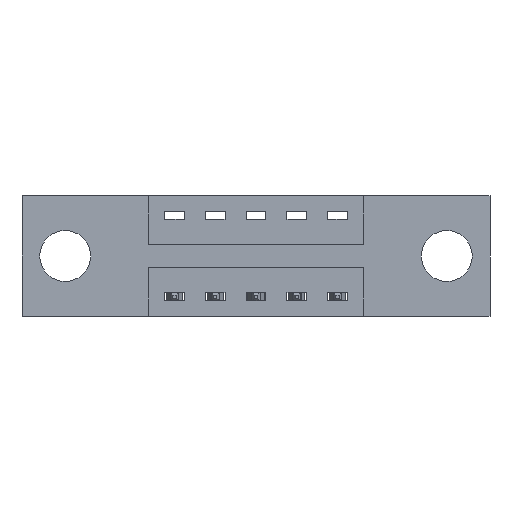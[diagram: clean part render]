
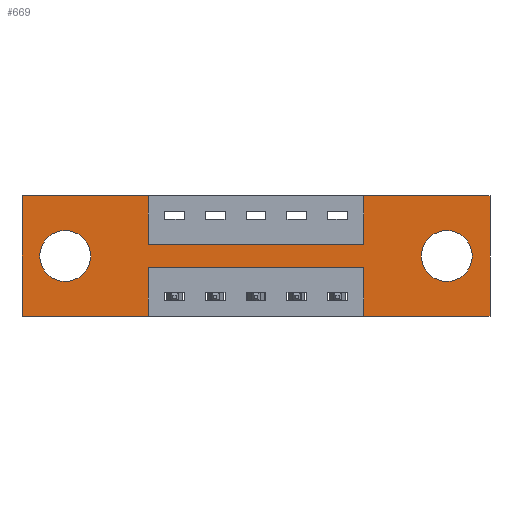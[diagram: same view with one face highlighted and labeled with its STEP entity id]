
A CAD part, front view. The second image highlights one B-rep face of the part: STEP entity #669.
In plain terms, the highlighted planar face has unit normal (0, -1, 0).
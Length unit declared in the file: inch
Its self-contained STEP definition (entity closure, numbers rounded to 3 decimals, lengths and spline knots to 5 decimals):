
#37 = EDGE_CURVE ( 'NONE', #6784, #6123, #3600, .T. ) ;
#101 = DIRECTION ( 'NONE',  ( 1., 0., 0. ) ) ;
#177 = CARTESIAN_POINT ( 'NONE',  ( 1.0475, 0., -0.37 ) ) ;
#225 = CARTESIAN_POINT ( 'NONE',  ( 0., 0., -0.37 ) ) ;
#285 = CARTESIAN_POINT ( 'NONE',  ( 1.0475, 0., -0.15 ) ) ;
#325 = CARTESIAN_POINT ( 'NONE',  ( 0.3875, 0., -0.37 ) ) ;
#384 = VECTOR ( 'NONE', #101, 39.37008 ) ;
#400 = ORIENTED_EDGE ( 'NONE', *, *, #2120, .T. ) ;
#424 = VERTEX_POINT ( 'NONE', #1286 ) ;
#450 = VERTEX_POINT ( 'NONE', #4074 ) ;
#461 = ORIENTED_EDGE ( 'NONE', *, *, #3175, .F. ) ;
#465 = CARTESIAN_POINT ( 'NONE',  ( 0., 0., 0. ) ) ;
#515 = CIRCLE ( 'NONE', #6175, 0.078 ) ;
#568 = CARTESIAN_POINT ( 'NONE',  ( 0., 0., 0. ) ) ;
#570 = EDGE_CURVE ( 'NONE', #2602, #4168, #8153, .T. ) ;
#615 = VERTEX_POINT ( 'NONE', #4347 ) ;
#669 = ADVANCED_FACE ( 'NONE', ( #4472, #1831, #4398 ), #5682, .T. ) ;
#696 = DIRECTION ( 'NONE',  ( -1., 0., 0. ) ) ;
#738 = CARTESIAN_POINT ( 'NONE',  ( 0., 0., -0.37 ) ) ;
#1146 = DIRECTION ( 'NONE',  ( 0., 0., 1. ) ) ;
#1165 = DIRECTION ( 'NONE',  ( 0., 0., 1. ) ) ;
#1175 = DIRECTION ( 'NONE',  ( 0., -1., 0. ) ) ;
#1286 = CARTESIAN_POINT ( 'NONE',  ( 0.3875, 0., -0.15 ) ) ;
#1293 = CARTESIAN_POINT ( 'NONE',  ( 0.3875, 0., -0.22 ) ) ;
#1321 = CARTESIAN_POINT ( 'NONE',  ( 1.435, 0., 0. ) ) ;
#1322 = ORIENTED_EDGE ( 'NONE', *, *, #5786, .F. ) ;
#1374 = CARTESIAN_POINT ( 'NONE',  ( 0.3875, 0., -0.15 ) ) ;
#1454 = CARTESIAN_POINT ( 'NONE',  ( 0.3875, 0., -0.37 ) ) ;
#1591 = EDGE_LOOP ( 'NONE', ( #4844, #400 ) ) ;
#1632 = EDGE_CURVE ( 'NONE', #4617, #7994, #2737, .T. ) ;
#1650 = VECTOR ( 'NONE', #3258, 39.37008 ) ;
#1731 = DIRECTION ( 'NONE',  ( 0., 0., -1. ) ) ;
#1772 = CARTESIAN_POINT ( 'NONE',  ( 1.0475, 0., 0. ) ) ;
#1787 = ORIENTED_EDGE ( 'NONE', *, *, #4769, .F. ) ;
#1831 = FACE_BOUND ( 'NONE', #1591, .T. ) ;
#1838 = ORIENTED_EDGE ( 'NONE', *, *, #6057, .F. ) ;
#1873 = CARTESIAN_POINT ( 'NONE',  ( 1.3025, 0., -0.107 ) ) ;
#1898 = DIRECTION ( 'NONE',  ( -1., 0., 0. ) ) ;
#1994 = DIRECTION ( 'NONE',  ( 0., 1., 0. ) ) ;
#2001 = CARTESIAN_POINT ( 'NONE',  ( 1.0475, 0., -0.37 ) ) ;
#2010 = EDGE_CURVE ( 'NONE', #5490, #6783, #7254, .T. ) ;
#2106 = ORIENTED_EDGE ( 'NONE', *, *, #6760, .F. ) ;
#2120 = EDGE_CURVE ( 'NONE', #6123, #6784, #515, .T. ) ;
#2315 = CARTESIAN_POINT ( 'NONE',  ( 1.435, 0., 0. ) ) ;
#2336 = VECTOR ( 'NONE', #696, 39.37008 ) ;
#2339 = CARTESIAN_POINT ( 'NONE',  ( 0.1325, 0., -0.263 ) ) ;
#2413 = ORIENTED_EDGE ( 'NONE', *, *, #570, .F. ) ;
#2414 = DIRECTION ( 'NONE',  ( 0., 1., 0. ) ) ;
#2449 = DIRECTION ( 'NONE',  ( 0., 0., -1. ) ) ;
#2491 = CIRCLE ( 'NONE', #8125, 0.078 ) ;
#2602 = VERTEX_POINT ( 'NONE', #225 ) ;
#2737 = CIRCLE ( 'NONE', #8519, 0.078 ) ;
#2891 = VERTEX_POINT ( 'NONE', #285 ) ;
#3007 = VECTOR ( 'NONE', #7327, 39.37008 ) ;
#3027 = CARTESIAN_POINT ( 'NONE',  ( 1.435, 0., -0.37 ) ) ;
#3170 = VERTEX_POINT ( 'NONE', #177 ) ;
#3175 = EDGE_CURVE ( 'NONE', #2891, #5490, #8078, .T. ) ;
#3258 = DIRECTION ( 'NONE',  ( 1., 0., 0. ) ) ;
#3360 = LINE ( 'NONE', #2001, #7794 ) ;
#3413 = CARTESIAN_POINT ( 'NONE',  ( 1.3025, 0., -0.185 ) ) ;
#3600 = CIRCLE ( 'NONE', #6176, 0.078 ) ;
#3632 = EDGE_CURVE ( 'NONE', #7407, #2602, #4011, .T. ) ;
#3702 = EDGE_CURVE ( 'NONE', #615, #450, #7265, .T. ) ;
#3720 = LINE ( 'NONE', #6319, #8499 ) ;
#3914 = ORIENTED_EDGE ( 'NONE', *, *, #4463, .T. ) ;
#3963 = VECTOR ( 'NONE', #1898, 39.37008 ) ;
#4011 = LINE ( 'NONE', #738, #2336 ) ;
#4074 = CARTESIAN_POINT ( 'NONE',  ( 0.3875, 0., -0.22 ) ) ;
#4155 = DIRECTION ( 'NONE',  ( 1., 0., 0. ) ) ;
#4168 = VERTEX_POINT ( 'NONE', #465 ) ;
#4294 = ORIENTED_EDGE ( 'NONE', *, *, #6850, .F. ) ;
#4347 = CARTESIAN_POINT ( 'NONE',  ( 1.0475, 0., -0.22 ) ) ;
#4398 = FACE_OUTER_BOUND ( 'NONE', #8339, .T. ) ;
#4416 = VECTOR ( 'NONE', #7435, 39.37008 ) ;
#4430 = ORIENTED_EDGE ( 'NONE', *, *, #7331, .F. ) ;
#4463 = EDGE_CURVE ( 'NONE', #7994, #4617, #2491, .T. ) ;
#4471 = LINE ( 'NONE', #1374, #384 ) ;
#4472 = FACE_BOUND ( 'NONE', #6003, .T. ) ;
#4601 = CARTESIAN_POINT ( 'NONE',  ( 0.1325, 0., -0.185 ) ) ;
#4617 = VERTEX_POINT ( 'NONE', #1873 ) ;
#4751 = DIRECTION ( 'NONE',  ( 0., 0., -1. ) ) ;
#4769 = EDGE_CURVE ( 'NONE', #424, #2891, #4471, .T. ) ;
#4844 = ORIENTED_EDGE ( 'NONE', *, *, #37, .T. ) ;
#4900 = CARTESIAN_POINT ( 'NONE',  ( 0., 0., 0. ) ) ;
#5022 = DIRECTION ( 'NONE',  ( 0., 0., -1. ) ) ;
#5117 = CARTESIAN_POINT ( 'NONE',  ( 0., 0., -0.37 ) ) ;
#5151 = CARTESIAN_POINT ( 'NONE',  ( 0., 0., -0.37 ) ) ;
#5192 = VECTOR ( 'NONE', #8380, 39.37008 ) ;
#5394 = DIRECTION ( 'NONE',  ( 0., 1., 0. ) ) ;
#5490 = VERTEX_POINT ( 'NONE', #1772 ) ;
#5618 = DIRECTION ( 'NONE',  ( -1., 0., 0. ) ) ;
#5682 = PLANE ( 'NONE',  #6476 ) ;
#5786 = EDGE_CURVE ( 'NONE', #4168, #6793, #6078, .T. ) ;
#5836 = CARTESIAN_POINT ( 'NONE',  ( 0.1325, 0., -0.107 ) ) ;
#5904 = VECTOR ( 'NONE', #4751, 39.37008 ) ;
#5906 = DIRECTION ( 'NONE',  ( 0., 0., -1. ) ) ;
#5981 = CARTESIAN_POINT ( 'NONE',  ( 0.1325, 0., -0.185 ) ) ;
#6003 = EDGE_LOOP ( 'NONE', ( #6939, #3914 ) ) ;
#6037 = VECTOR ( 'NONE', #5618, 39.37008 ) ;
#6057 = EDGE_CURVE ( 'NONE', #3170, #615, #3360, .T. ) ;
#6078 = LINE ( 'NONE', #6917, #8293 ) ;
#6123 = VERTEX_POINT ( 'NONE', #2339 ) ;
#6146 = VERTEX_POINT ( 'NONE', #3027 ) ;
#6175 = AXIS2_PLACEMENT_3D ( 'NONE', #5981, #1994, #7908 ) ;
#6176 = AXIS2_PLACEMENT_3D ( 'NONE', #4601, #7243, #1165 ) ;
#6319 = CARTESIAN_POINT ( 'NONE',  ( 0.3875, 0., 0. ) ) ;
#6326 = CARTESIAN_POINT ( 'NONE',  ( 1.3025, 0., -0.185 ) ) ;
#6430 = ORIENTED_EDGE ( 'NONE', *, *, #2010, .F. ) ;
#6476 = AXIS2_PLACEMENT_3D ( 'NONE', #5117, #1175, #1731 ) ;
#6760 = EDGE_CURVE ( 'NONE', #6146, #3170, #8443, .T. ) ;
#6783 = VERTEX_POINT ( 'NONE', #1321 ) ;
#6784 = VERTEX_POINT ( 'NONE', #5836 ) ;
#6789 = ORIENTED_EDGE ( 'NONE', *, *, #3702, .F. ) ;
#6793 = VERTEX_POINT ( 'NONE', #7214 ) ;
#6796 = LINE ( 'NONE', #1454, #5904 ) ;
#6850 = EDGE_CURVE ( 'NONE', #6793, #424, #3720, .T. ) ;
#6880 = ORIENTED_EDGE ( 'NONE', *, *, #8160, .F. ) ;
#6917 = CARTESIAN_POINT ( 'NONE',  ( 0., 0., 0. ) ) ;
#6939 = ORIENTED_EDGE ( 'NONE', *, *, #1632, .T. ) ;
#7214 = CARTESIAN_POINT ( 'NONE',  ( 0.3875, 0., 0. ) ) ;
#7243 = DIRECTION ( 'NONE',  ( 0., 1., 0. ) ) ;
#7254 = LINE ( 'NONE', #568, #1650 ) ;
#7265 = LINE ( 'NONE', #1293, #6037 ) ;
#7327 = DIRECTION ( 'NONE',  ( 0., 0., 1. ) ) ;
#7331 = EDGE_CURVE ( 'NONE', #6783, #6146, #8303, .T. ) ;
#7407 = VERTEX_POINT ( 'NONE', #325 ) ;
#7435 = DIRECTION ( 'NONE',  ( 0., 0., 1. ) ) ;
#7454 = CARTESIAN_POINT ( 'NONE',  ( 1.0475, 0., 0. ) ) ;
#7794 = VECTOR ( 'NONE', #1146, 39.37008 ) ;
#7908 = DIRECTION ( 'NONE',  ( 0., 0., 1. ) ) ;
#7923 = ORIENTED_EDGE ( 'NONE', *, *, #3632, .F. ) ;
#7994 = VERTEX_POINT ( 'NONE', #8269 ) ;
#8078 = LINE ( 'NONE', #7454, #3007 ) ;
#8125 = AXIS2_PLACEMENT_3D ( 'NONE', #3413, #5394, #5906 ) ;
#8153 = LINE ( 'NONE', #4900, #4416 ) ;
#8160 = EDGE_CURVE ( 'NONE', #450, #7407, #6796, .T. ) ;
#8269 = CARTESIAN_POINT ( 'NONE',  ( 1.3025, 0., -0.263 ) ) ;
#8293 = VECTOR ( 'NONE', #4155, 39.37008 ) ;
#8303 = LINE ( 'NONE', #2315, #5192 ) ;
#8339 = EDGE_LOOP ( 'NONE', ( #6880, #6789, #1838, #2106, #4430, #6430, #461, #1787, #4294, #1322, #2413, #7923 ) ) ;
#8380 = DIRECTION ( 'NONE',  ( 0., 0., -1. ) ) ;
#8443 = LINE ( 'NONE', #5151, #3963 ) ;
#8499 = VECTOR ( 'NONE', #2449, 39.37008 ) ;
#8519 = AXIS2_PLACEMENT_3D ( 'NONE', #6326, #2414, #5022 ) ;
